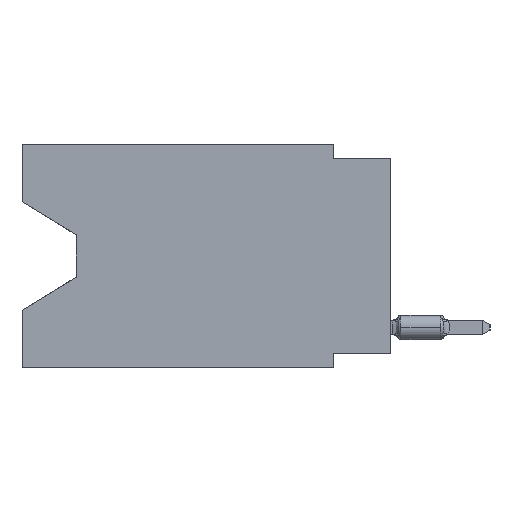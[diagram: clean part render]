
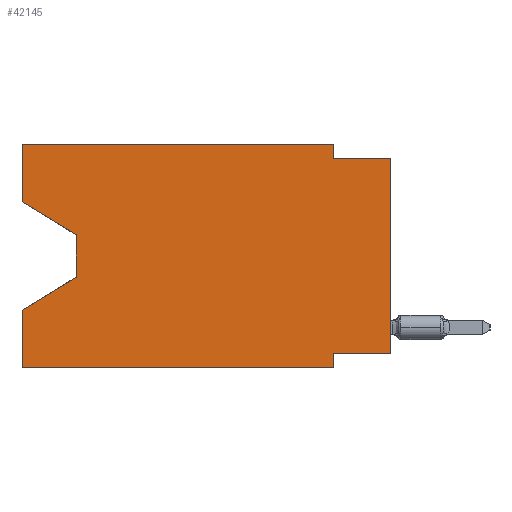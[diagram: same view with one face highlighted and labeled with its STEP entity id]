
A CAD part, left-side view. The second image highlights one B-rep face of the part: STEP entity #42145.
In plain terms, the highlighted planar face has unit normal (-1, 0, 0).
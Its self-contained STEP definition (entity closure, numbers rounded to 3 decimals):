
#479 = VERTEX_POINT ( 'NONE', #42642 ) ;
#657 = ORIENTED_EDGE ( 'NONE', *, *, #1244, .T. ) ;
#1244 = EDGE_CURVE ( 'NONE', #16225, #479, #39093, .T. ) ;
#1570 = LINE ( 'NONE', #27345, #5773 ) ;
#1996 = CARTESIAN_POINT ( 'NONE',  ( 0., 16.383, 0. ) ) ;
#2108 = CARTESIAN_POINT ( 'NONE',  ( 0., 0., -0.635 ) ) ;
#2570 = DIRECTION ( 'NONE',  ( 0., -1., 0. ) ) ;
#3630 = VERTEX_POINT ( 'NONE', #39584 ) ;
#3832 = CARTESIAN_POINT ( 'NONE',  ( 0., 16.383, 0. ) ) ;
#4133 = ORIENTED_EDGE ( 'NONE', *, *, #30374, .F. ) ;
#5773 = VECTOR ( 'NONE', #2570, 1000. ) ;
#6766 = VECTOR ( 'NONE', #33477, 1000. ) ;
#7709 = DIRECTION ( 'NONE',  ( 0., 0., 1. ) ) ;
#7982 = DIRECTION ( 'NONE',  ( 0., 0., 1. ) ) ;
#8345 = EDGE_CURVE ( 'NONE', #63164, #479, #21872, .T. ) ;
#8351 = PLANE ( 'NONE',  #38391 ) ;
#8637 = LINE ( 'NONE', #44442, #36490 ) ;
#8676 = FACE_OUTER_BOUND ( 'NONE', #14285, .T. ) ;
#9566 = VERTEX_POINT ( 'NONE', #29768 ) ;
#9764 = CARTESIAN_POINT ( 'NONE',  ( 0., 2.54, 0. ) ) ;
#10353 = ORIENTED_EDGE ( 'NONE', *, *, #53533, .T. ) ;
#12382 = LINE ( 'NONE', #1996, #51677 ) ;
#12514 = EDGE_CURVE ( 'NONE', #63538, #58719, #43192, .T. ) ;
#13125 = VECTOR ( 'NONE', #50014, 1000. ) ;
#13210 = CARTESIAN_POINT ( 'NONE',  ( 0., 0., -9.271 ) ) ;
#14285 = EDGE_LOOP ( 'NONE', ( #10353, #46467, #47803, #47012, #43802, #4133, #62162, #657, #65534, #23648, #20250, #44012 ) ) ;
#14407 = LINE ( 'NONE', #45193, #22759 ) ;
#16225 = VERTEX_POINT ( 'NONE', #13210 ) ;
#18024 = CARTESIAN_POINT ( 'NONE',  ( 0., 13.97, -4.013 ) ) ;
#18100 = CARTESIAN_POINT ( 'NONE',  ( 0., 16.383, -7.36 ) ) ;
#19065 = EDGE_CURVE ( 'NONE', #53240, #58361, #12382, .T. ) ;
#19203 = CARTESIAN_POINT ( 'NONE',  ( 0., 2.54, 0. ) ) ;
#20147 = CARTESIAN_POINT ( 'NONE',  ( 0., 16.383, -9.906 ) ) ;
#20250 = ORIENTED_EDGE ( 'NONE', *, *, #57567, .F. ) ;
#21872 = LINE ( 'NONE', #2108, #34058 ) ;
#22069 = VERTEX_POINT ( 'NONE', #9764 ) ;
#22759 = VECTOR ( 'NONE', #39838, 1000. ) ;
#23348 = CARTESIAN_POINT ( 'NONE',  ( 0., 0., 0. ) ) ;
#23648 = ORIENTED_EDGE ( 'NONE', *, *, #36980, .F. ) ;
#24284 = CARTESIAN_POINT ( 'NONE',  ( 0., 2.54, -0.635 ) ) ;
#26919 = EDGE_CURVE ( 'NONE', #53240, #3630, #1570, .T. ) ;
#27219 = DIRECTION ( 'NONE',  ( 0., -1., 0. ) ) ;
#27345 = CARTESIAN_POINT ( 'NONE',  ( 0., 16.383, -9.906 ) ) ;
#27470 = VERTEX_POINT ( 'NONE', #65893 ) ;
#28748 = DIRECTION ( 'NONE',  ( 1., 0., 0. ) ) ;
#29029 = DIRECTION ( 'NONE',  ( 0., 0.855, -0.519 ) ) ;
#29768 = CARTESIAN_POINT ( 'NONE',  ( 0., 13.97, -5.893 ) ) ;
#30374 = EDGE_CURVE ( 'NONE', #27470, #3630, #41974, .T. ) ;
#31242 = CARTESIAN_POINT ( 'NONE',  ( 0., 16.383, 0. ) ) ;
#31648 = VECTOR ( 'NONE', #40735, 1000. ) ;
#31840 = EDGE_CURVE ( 'NONE', #16225, #27470, #50486, .T. ) ;
#32795 = DIRECTION ( 'NONE',  ( 0., 0., 1. ) ) ;
#33134 = CARTESIAN_POINT ( 'NONE',  ( 0., 16.383, 0. ) ) ;
#33477 = DIRECTION ( 'NONE',  ( 0., -0.855, -0.519 ) ) ;
#34058 = VECTOR ( 'NONE', #27219, 1000. ) ;
#36490 = VECTOR ( 'NONE', #29029, 1000. ) ;
#36980 = EDGE_CURVE ( 'NONE', #22069, #63164, #60055, .T. ) ;
#38391 = AXIS2_PLACEMENT_3D ( 'NONE', #39144, #28748, #49193 ) ;
#39093 = LINE ( 'NONE', #23348, #48261 ) ;
#39144 = CARTESIAN_POINT ( 'NONE',  ( 0., 16.383, 0. ) ) ;
#39165 = VECTOR ( 'NONE', #52056, 1000. ) ;
#39584 = CARTESIAN_POINT ( 'NONE',  ( 0., 2.54, -9.906 ) ) ;
#39838 = DIRECTION ( 'NONE',  ( 0., 0., -1. ) ) ;
#40275 = CARTESIAN_POINT ( 'NONE',  ( 0., 16.383, -2.546 ) ) ;
#40735 = DIRECTION ( 'NONE',  ( 0., 1., 0. ) ) ;
#41974 = LINE ( 'NONE', #57403, #39165 ) ;
#42145 = ADVANCED_FACE ( 'NONE', ( #8676 ), #8351, .F. ) ;
#42642 = CARTESIAN_POINT ( 'NONE',  ( 0., 0., -0.635 ) ) ;
#43192 = LINE ( 'NONE', #33134, #44784 ) ;
#43802 = ORIENTED_EDGE ( 'NONE', *, *, #26919, .T. ) ;
#44012 = ORIENTED_EDGE ( 'NONE', *, *, #12514, .F. ) ;
#44192 = LINE ( 'NONE', #49219, #6766 ) ;
#44442 = CARTESIAN_POINT ( 'NONE',  ( 0., 13.97, -5.893 ) ) ;
#44784 = VECTOR ( 'NONE', #7709, 1000. ) ;
#45193 = CARTESIAN_POINT ( 'NONE',  ( 0., 13.97, -4.013 ) ) ;
#46467 = ORIENTED_EDGE ( 'NONE', *, *, #61157, .T. ) ;
#47012 = ORIENTED_EDGE ( 'NONE', *, *, #19065, .F. ) ;
#47803 = ORIENTED_EDGE ( 'NONE', *, *, #60364, .T. ) ;
#48261 = VECTOR ( 'NONE', #7982, 1000. ) ;
#49193 = DIRECTION ( 'NONE',  ( 0., 0., -1. ) ) ;
#49219 = CARTESIAN_POINT ( 'NONE',  ( 0., 16.383, -2.546 ) ) ;
#50014 = DIRECTION ( 'NONE',  ( 0., 0., -1. ) ) ;
#50486 = LINE ( 'NONE', #66189, #31648 ) ;
#51369 = LINE ( 'NONE', #31242, #54000 ) ;
#51677 = VECTOR ( 'NONE', #32795, 1000. ) ;
#52056 = DIRECTION ( 'NONE',  ( 0., 0., -1. ) ) ;
#53240 = VERTEX_POINT ( 'NONE', #20147 ) ;
#53533 = EDGE_CURVE ( 'NONE', #63538, #60301, #44192, .T. ) ;
#54000 = VECTOR ( 'NONE', #65765, 1000. ) ;
#57403 = CARTESIAN_POINT ( 'NONE',  ( 0., 2.54, -9.906 ) ) ;
#57567 = EDGE_CURVE ( 'NONE', #58719, #22069, #51369, .T. ) ;
#58361 = VERTEX_POINT ( 'NONE', #18100 ) ;
#58719 = VERTEX_POINT ( 'NONE', #3832 ) ;
#60055 = LINE ( 'NONE', #19203, #13125 ) ;
#60301 = VERTEX_POINT ( 'NONE', #18024 ) ;
#60364 = EDGE_CURVE ( 'NONE', #9566, #58361, #8637, .T. ) ;
#61157 = EDGE_CURVE ( 'NONE', #60301, #9566, #14407, .T. ) ;
#62162 = ORIENTED_EDGE ( 'NONE', *, *, #31840, .F. ) ;
#63164 = VERTEX_POINT ( 'NONE', #24284 ) ;
#63538 = VERTEX_POINT ( 'NONE', #40275 ) ;
#65534 = ORIENTED_EDGE ( 'NONE', *, *, #8345, .F. ) ;
#65765 = DIRECTION ( 'NONE',  ( 0., -1., 0. ) ) ;
#65893 = CARTESIAN_POINT ( 'NONE',  ( 0., 2.54, -9.271 ) ) ;
#66189 = CARTESIAN_POINT ( 'NONE',  ( 0., 0., -9.271 ) ) ;
